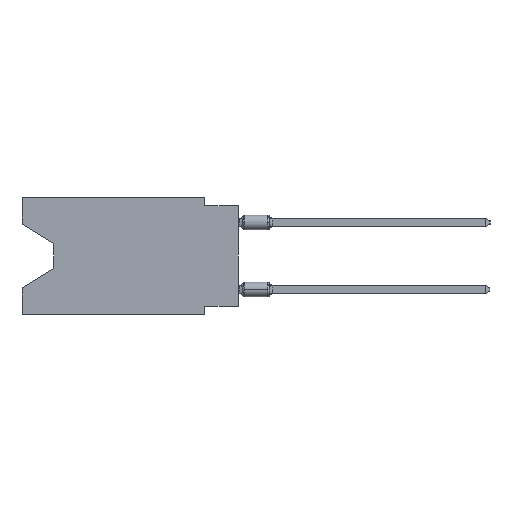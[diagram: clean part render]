
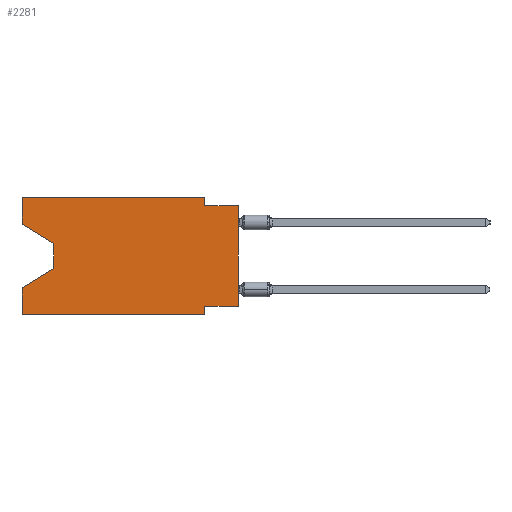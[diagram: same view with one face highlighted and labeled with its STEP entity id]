
A CAD part, left-side view. The second image highlights one B-rep face of the part: STEP entity #2281.
In plain terms, the highlighted planar face has unit normal (-1, 0, 0).
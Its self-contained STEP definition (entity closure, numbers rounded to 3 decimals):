
#5 = ORIENTED_EDGE ( 'NONE', *, *, #10997, .F. ) ;
#296 = EDGE_CURVE ( 'NONE', #10917, #2689, #14627, .T. ) ;
#471 = VERTEX_POINT ( 'NONE', #2518 ) ;
#523 = ORIENTED_EDGE ( 'NONE', *, *, #5378, .T. ) ;
#875 = VERTEX_POINT ( 'NONE', #3458 ) ;
#1165 = CARTESIAN_POINT ( 'NONE',  ( 0., 16.383, -2.038 ) ) ;
#1277 = CARTESIAN_POINT ( 'NONE',  ( 0., 16.383, -8.89 ) ) ;
#1378 = VECTOR ( 'NONE', #3224, 1000. ) ;
#1425 = VECTOR ( 'NONE', #9890, 1000. ) ;
#2031 = ORIENTED_EDGE ( 'NONE', *, *, #8291, .T. ) ;
#2123 = EDGE_CURVE ( 'NONE', #5088, #7323, #8215, .T. ) ;
#2281 = ADVANCED_FACE ( 'NONE', ( #12997 ), #7318, .F. ) ;
#2290 = LINE ( 'NONE', #14095, #11138 ) ;
#2518 = CARTESIAN_POINT ( 'NONE',  ( 0., 0., -0.635 ) ) ;
#2523 = ORIENTED_EDGE ( 'NONE', *, *, #9462, .F. ) ;
#2536 = DIRECTION ( 'NONE',  ( 0., 0., 1. ) ) ;
#2689 = VERTEX_POINT ( 'NONE', #10813 ) ;
#2978 = EDGE_CURVE ( 'NONE', #6664, #14885, #2290, .T. ) ;
#3021 = CARTESIAN_POINT ( 'NONE',  ( 0., 16.383, -6.852 ) ) ;
#3194 = LINE ( 'NONE', #5251, #1425 ) ;
#3224 = DIRECTION ( 'NONE',  ( 0., -0.855, -0.519 ) ) ;
#3252 = ORIENTED_EDGE ( 'NONE', *, *, #5344, .F. ) ;
#3407 = DIRECTION ( 'NONE',  ( 0., -1., 0. ) ) ;
#3418 = ORIENTED_EDGE ( 'NONE', *, *, #6611, .F. ) ;
#3444 = DIRECTION ( 'NONE',  ( 0., 0., 1. ) ) ;
#3458 = CARTESIAN_POINT ( 'NONE',  ( 0., 16.383, -2.038 ) ) ;
#3894 = EDGE_CURVE ( 'NONE', #6170, #7323, #13590, .T. ) ;
#4041 = DIRECTION ( 'NONE',  ( 0., -1., 0. ) ) ;
#4194 = CARTESIAN_POINT ( 'NONE',  ( 0., 16.383, 0. ) ) ;
#4287 = EDGE_LOOP ( 'NONE', ( #7810, #523, #13992, #7377, #10492, #8434, #5, #2031, #2523, #3252, #7681, #3418 ) ) ;
#4438 = VERTEX_POINT ( 'NONE', #5931 ) ;
#4576 = DIRECTION ( 'NONE',  ( 0., 0.855, -0.519 ) ) ;
#4596 = LINE ( 'NONE', #1165, #1378 ) ;
#4648 = CARTESIAN_POINT ( 'NONE',  ( 0., 2.54, -0.635 ) ) ;
#5088 = VERTEX_POINT ( 'NONE', #11541 ) ;
#5251 = CARTESIAN_POINT ( 'NONE',  ( 0., 0., -0.635 ) ) ;
#5344 = EDGE_CURVE ( 'NONE', #2689, #9253, #7538, .T. ) ;
#5378 = EDGE_CURVE ( 'NONE', #7877, #6664, #10014, .T. ) ;
#5931 = CARTESIAN_POINT ( 'NONE',  ( 0., 0., -8.255 ) ) ;
#6170 = VERTEX_POINT ( 'NONE', #11104 ) ;
#6232 = VECTOR ( 'NONE', #13521, 1000. ) ;
#6322 = LINE ( 'NONE', #10941, #7482 ) ;
#6611 = EDGE_CURVE ( 'NONE', #875, #10917, #6322, .T. ) ;
#6664 = VERTEX_POINT ( 'NONE', #11393 ) ;
#6718 = VECTOR ( 'NONE', #2536, 1000. ) ;
#6776 = CARTESIAN_POINT ( 'NONE',  ( 0., 13.97, -3.505 ) ) ;
#6943 = VECTOR ( 'NONE', #7668, 1000. ) ;
#7235 = CARTESIAN_POINT ( 'NONE',  ( 0., 16.383, 0. ) ) ;
#7318 = PLANE ( 'NONE',  #11593 ) ;
#7323 = VERTEX_POINT ( 'NONE', #8176 ) ;
#7377 = ORIENTED_EDGE ( 'NONE', *, *, #15041, .F. ) ;
#7482 = VECTOR ( 'NONE', #14442, 1000. ) ;
#7538 = LINE ( 'NONE', #8745, #12533 ) ;
#7668 = DIRECTION ( 'NONE',  ( 0., 0., -1. ) ) ;
#7681 = ORIENTED_EDGE ( 'NONE', *, *, #296, .F. ) ;
#7810 = ORIENTED_EDGE ( 'NONE', *, *, #10399, .T. ) ;
#7877 = VERTEX_POINT ( 'NONE', #6776 ) ;
#7882 = CARTESIAN_POINT ( 'NONE',  ( 0., 2.54, -8.89 ) ) ;
#8176 = CARTESIAN_POINT ( 'NONE',  ( 0., 2.54, -8.89 ) ) ;
#8215 = LINE ( 'NONE', #1277, #11841 ) ;
#8261 = LINE ( 'NONE', #12959, #6718 ) ;
#8291 = EDGE_CURVE ( 'NONE', #4438, #471, #9027, .T. ) ;
#8434 = ORIENTED_EDGE ( 'NONE', *, *, #3894, .F. ) ;
#8745 = CARTESIAN_POINT ( 'NONE',  ( 0., 2.54, 0. ) ) ;
#8887 = CARTESIAN_POINT ( 'NONE',  ( 0., 13.97, -3.505 ) ) ;
#9027 = LINE ( 'NONE', #13875, #11118 ) ;
#9075 = CARTESIAN_POINT ( 'NONE',  ( 0., 16.383, 0. ) ) ;
#9253 = VERTEX_POINT ( 'NONE', #4648 ) ;
#9462 = EDGE_CURVE ( 'NONE', #9253, #471, #3194, .T. ) ;
#9723 = DIRECTION ( 'NONE',  ( 0., 0., -1. ) ) ;
#9727 = DIRECTION ( 'NONE',  ( 0., 0., -1. ) ) ;
#9890 = DIRECTION ( 'NONE',  ( 0., -1., 0. ) ) ;
#10014 = LINE ( 'NONE', #8887, #6232 ) ;
#10399 = EDGE_CURVE ( 'NONE', #875, #7877, #4596, .T. ) ;
#10428 = CARTESIAN_POINT ( 'NONE',  ( 0., 0., -8.255 ) ) ;
#10492 = ORIENTED_EDGE ( 'NONE', *, *, #2123, .T. ) ;
#10495 = LINE ( 'NONE', #10428, #11589 ) ;
#10813 = CARTESIAN_POINT ( 'NONE',  ( 0., 2.54, 0. ) ) ;
#10895 = VECTOR ( 'NONE', #4041, 1000. ) ;
#10917 = VERTEX_POINT ( 'NONE', #9075 ) ;
#10941 = CARTESIAN_POINT ( 'NONE',  ( 0., 16.383, 0. ) ) ;
#10997 = EDGE_CURVE ( 'NONE', #4438, #6170, #10495, .T. ) ;
#11104 = CARTESIAN_POINT ( 'NONE',  ( 0., 2.54, -8.255 ) ) ;
#11118 = VECTOR ( 'NONE', #3444, 1000. ) ;
#11138 = VECTOR ( 'NONE', #4576, 1000. ) ;
#11393 = CARTESIAN_POINT ( 'NONE',  ( 0., 13.97, -5.385 ) ) ;
#11541 = CARTESIAN_POINT ( 'NONE',  ( 0., 16.383, -8.89 ) ) ;
#11589 = VECTOR ( 'NONE', #14010, 1000. ) ;
#11593 = AXIS2_PLACEMENT_3D ( 'NONE', #7235, #11854, #9727 ) ;
#11841 = VECTOR ( 'NONE', #3407, 1000. ) ;
#11854 = DIRECTION ( 'NONE',  ( 1., 0., 0. ) ) ;
#12533 = VECTOR ( 'NONE', #9723, 1000. ) ;
#12959 = CARTESIAN_POINT ( 'NONE',  ( 0., 16.383, 0. ) ) ;
#12997 = FACE_OUTER_BOUND ( 'NONE', #4287, .T. ) ;
#13521 = DIRECTION ( 'NONE',  ( 0., 0., -1. ) ) ;
#13590 = LINE ( 'NONE', #7882, #6943 ) ;
#13875 = CARTESIAN_POINT ( 'NONE',  ( 0., 0., 0. ) ) ;
#13992 = ORIENTED_EDGE ( 'NONE', *, *, #2978, .T. ) ;
#14010 = DIRECTION ( 'NONE',  ( 0., 1., 0. ) ) ;
#14095 = CARTESIAN_POINT ( 'NONE',  ( 0., 13.97, -5.385 ) ) ;
#14442 = DIRECTION ( 'NONE',  ( 0., 0., 1. ) ) ;
#14627 = LINE ( 'NONE', #4194, #10895 ) ;
#14885 = VERTEX_POINT ( 'NONE', #3021 ) ;
#15041 = EDGE_CURVE ( 'NONE', #5088, #14885, #8261, .T. ) ;
